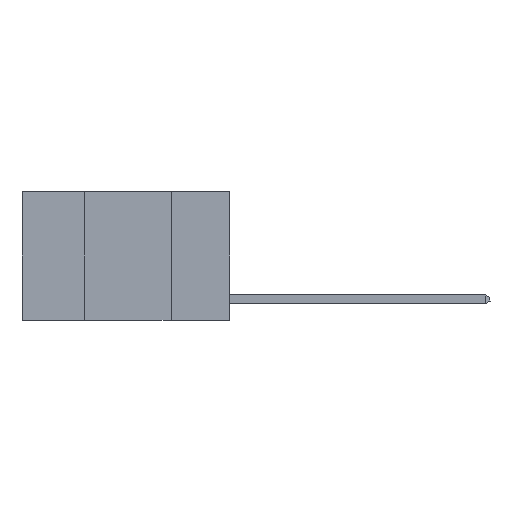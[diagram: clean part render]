
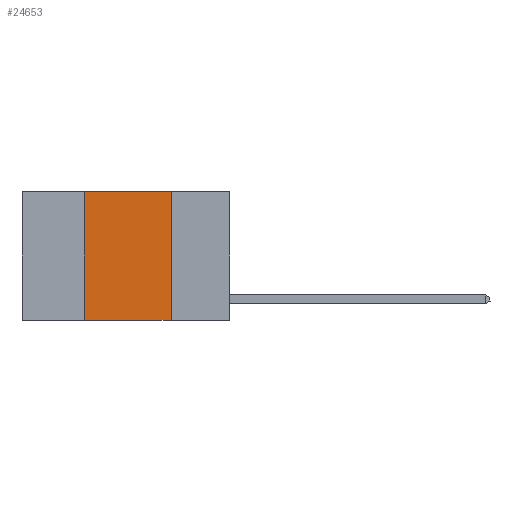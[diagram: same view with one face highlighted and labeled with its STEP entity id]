
A CAD part, left-side view. The second image highlights one B-rep face of the part: STEP entity #24653.
In plain terms, the highlighted planar face has unit normal (-1, 0, 0).
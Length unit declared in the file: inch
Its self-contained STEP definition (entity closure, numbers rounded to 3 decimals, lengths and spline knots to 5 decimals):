
#4066 = VERTEX_POINT ( 'NONE', #13897 ) ;
#4527 = CARTESIAN_POINT ( 'NONE',  ( 0., 0.6, -0.37 ) ) ;
#6517 = DIRECTION ( 'NONE',  ( 1., 0., 0. ) ) ;
#6585 = EDGE_CURVE ( 'NONE', #16704, #7494, #21440, .T. ) ;
#7494 = VERTEX_POINT ( 'NONE', #27252 ) ;
#7675 = VECTOR ( 'NONE', #13346, 39.37008 ) ;
#7833 = VECTOR ( 'NONE', #27391, 39.37008 ) ;
#8745 = VECTOR ( 'NONE', #22566, 39.37008 ) ;
#9015 = LINE ( 'NONE', #12112, #8745 ) ;
#9265 = AXIS2_PLACEMENT_3D ( 'NONE', #19263, #6517, #23572 ) ;
#9679 = ORIENTED_EDGE ( 'NONE', *, *, #21239, .F. ) ;
#10089 = CARTESIAN_POINT ( 'NONE',  ( 0., 0.6, 0. ) ) ;
#10739 = FACE_OUTER_BOUND ( 'NONE', #18476, .T. ) ;
#11846 = EDGE_CURVE ( 'NONE', #4066, #7494, #9015, .T. ) ;
#12046 = LINE ( 'NONE', #10089, #7833 ) ;
#12112 = CARTESIAN_POINT ( 'NONE',  ( 0., 0.17, 0. ) ) ;
#12378 = VERTEX_POINT ( 'NONE', #14038 ) ;
#13346 = DIRECTION ( 'NONE',  ( 0., -1., 0. ) ) ;
#13897 = CARTESIAN_POINT ( 'NONE',  ( 0., 0.17, 0. ) ) ;
#14038 = CARTESIAN_POINT ( 'NONE',  ( 0., 0.42, 0. ) ) ;
#14372 = ORIENTED_EDGE ( 'NONE', *, *, #24016, .F. ) ;
#15076 = PLANE ( 'NONE',  #9265 ) ;
#16579 = ORIENTED_EDGE ( 'NONE', *, *, #6585, .T. ) ;
#16704 = VERTEX_POINT ( 'NONE', #17918 ) ;
#17918 = CARTESIAN_POINT ( 'NONE',  ( 0., 0.42, -0.37 ) ) ;
#18476 = EDGE_LOOP ( 'NONE', ( #21469, #14372, #9679, #16579 ) ) ;
#19263 = CARTESIAN_POINT ( 'NONE',  ( 0., 0.6, 0. ) ) ;
#21239 = EDGE_CURVE ( 'NONE', #16704, #12378, #26818, .T. ) ;
#21440 = LINE ( 'NONE', #4527, #7675 ) ;
#21469 = ORIENTED_EDGE ( 'NONE', *, *, #11846, .F. ) ;
#22566 = DIRECTION ( 'NONE',  ( 0., 0., -1. ) ) ;
#22615 = CARTESIAN_POINT ( 'NONE',  ( 0., 0.42, 0. ) ) ;
#22873 = VECTOR ( 'NONE', #25816, 39.37008 ) ;
#23572 = DIRECTION ( 'NONE',  ( 0., 0., -1. ) ) ;
#24016 = EDGE_CURVE ( 'NONE', #12378, #4066, #12046, .T. ) ;
#24653 = ADVANCED_FACE ( 'NONE', ( #10739 ), #15076, .F. ) ;
#25816 = DIRECTION ( 'NONE',  ( 0., 0., 1. ) ) ;
#26818 = LINE ( 'NONE', #22615, #22873 ) ;
#27252 = CARTESIAN_POINT ( 'NONE',  ( 0., 0.17, -0.37 ) ) ;
#27391 = DIRECTION ( 'NONE',  ( 0., -1., 0. ) ) ;
